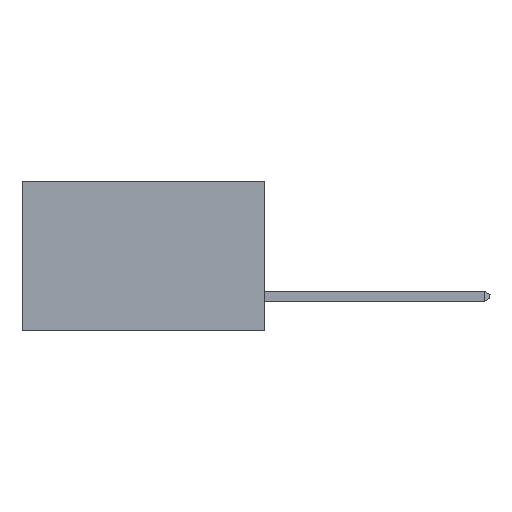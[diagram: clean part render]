
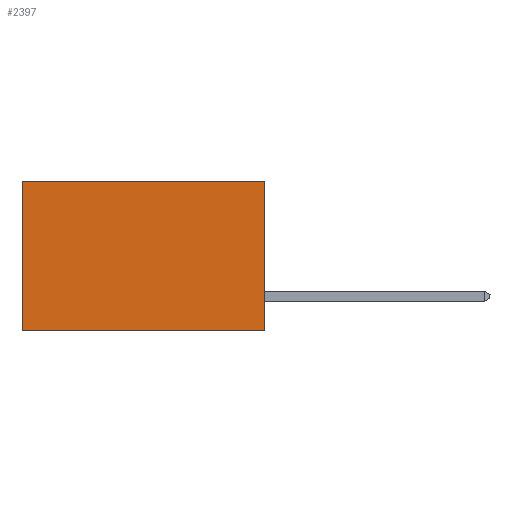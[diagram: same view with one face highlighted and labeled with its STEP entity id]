
A CAD part, left-side view. The second image highlights one B-rep face of the part: STEP entity #2397.
In plain terms, the highlighted planar face has unit normal (-1, 0, 0).
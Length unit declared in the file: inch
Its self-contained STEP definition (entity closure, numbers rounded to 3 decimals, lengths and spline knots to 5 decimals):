
#36 = VECTOR ( 'NONE', #5215, 39.37008 ) ;
#929 = AXIS2_PLACEMENT_3D ( 'NONE', #4730, #1606, #13103 ) ;
#1290 = EDGE_CURVE ( 'NONE', #3796, #7128, #8102, .T. ) ;
#1606 = DIRECTION ( 'NONE',  ( 1., 0., 0. ) ) ;
#1847 = VECTOR ( 'NONE', #2280, 39.37008 ) ;
#2280 = DIRECTION ( 'NONE',  ( 0., 0., -1. ) ) ;
#2397 = ADVANCED_FACE ( 'NONE', ( #4625 ), #4918, .F. ) ;
#3761 = VERTEX_POINT ( 'NONE', #7481 ) ;
#3796 = VERTEX_POINT ( 'NONE', #4490 ) ;
#4490 = CARTESIAN_POINT ( 'NONE',  ( 0.298, 0., -0.37 ) ) ;
#4625 = FACE_OUTER_BOUND ( 'NONE', #9137, .T. ) ;
#4730 = CARTESIAN_POINT ( 'NONE',  ( 0.298, 0., 0. ) ) ;
#4918 = PLANE ( 'NONE',  #929 ) ;
#5215 = DIRECTION ( 'NONE',  ( 0., 0., -1. ) ) ;
#5362 = CARTESIAN_POINT ( 'NONE',  ( 0.298, 0.6, 0. ) ) ;
#5507 = EDGE_CURVE ( 'NONE', #3761, #3796, #11487, .T. ) ;
#6851 = VECTOR ( 'NONE', #12834, 39.37008 ) ;
#7128 = VERTEX_POINT ( 'NONE', #7643 ) ;
#7381 = CARTESIAN_POINT ( 'NONE',  ( 0.298, 0., 0. ) ) ;
#7481 = CARTESIAN_POINT ( 'NONE',  ( 0.298, 0., 0. ) ) ;
#7643 = CARTESIAN_POINT ( 'NONE',  ( 0.298, 0.6, -0.37 ) ) ;
#8102 = LINE ( 'NONE', #10419, #6851 ) ;
#8740 = DIRECTION ( 'NONE',  ( 0., 1., 0. ) ) ;
#9117 = LINE ( 'NONE', #7381, #10576 ) ;
#9137 = EDGE_LOOP ( 'NONE', ( #10872, #9746, #12869, #13947 ) ) ;
#9225 = CARTESIAN_POINT ( 'NONE',  ( 0.298, 0., 0. ) ) ;
#9746 = ORIENTED_EDGE ( 'NONE', *, *, #1290, .F. ) ;
#10419 = CARTESIAN_POINT ( 'NONE',  ( 0.298, 0., -0.37 ) ) ;
#10576 = VECTOR ( 'NONE', #8740, 39.37008 ) ;
#10790 = VERTEX_POINT ( 'NONE', #13715 ) ;
#10872 = ORIENTED_EDGE ( 'NONE', *, *, #12571, .T. ) ;
#11487 = LINE ( 'NONE', #9225, #1847 ) ;
#12121 = EDGE_CURVE ( 'NONE', #3761, #10790, #9117, .T. ) ;
#12571 = EDGE_CURVE ( 'NONE', #10790, #7128, #12727, .T. ) ;
#12727 = LINE ( 'NONE', #5362, #36 ) ;
#12834 = DIRECTION ( 'NONE',  ( 0., 1., 0. ) ) ;
#12869 = ORIENTED_EDGE ( 'NONE', *, *, #5507, .F. ) ;
#13103 = DIRECTION ( 'NONE',  ( 0., 0., -1. ) ) ;
#13715 = CARTESIAN_POINT ( 'NONE',  ( 0.298, 0.6, 0. ) ) ;
#13947 = ORIENTED_EDGE ( 'NONE', *, *, #12121, .T. ) ;
